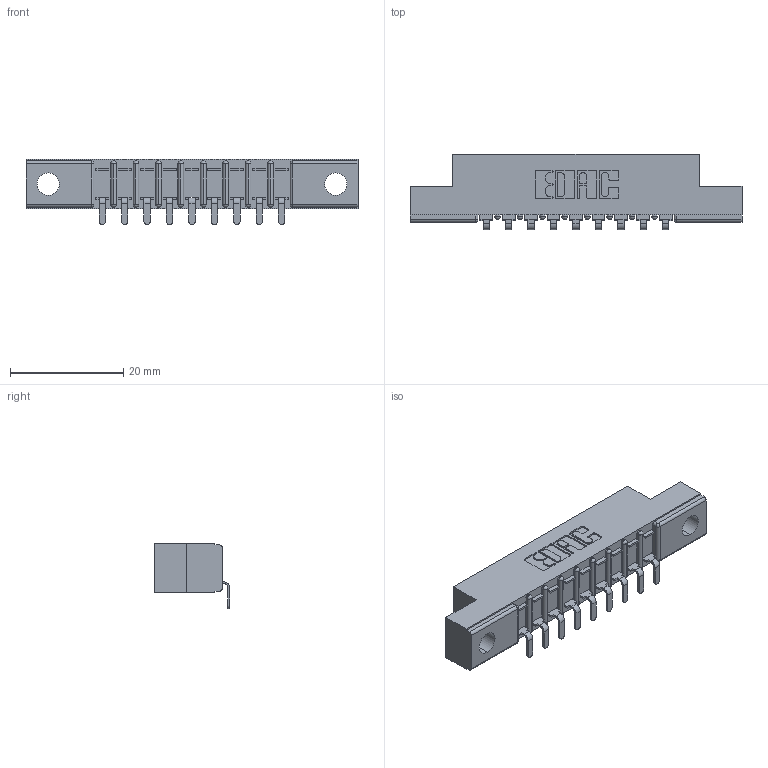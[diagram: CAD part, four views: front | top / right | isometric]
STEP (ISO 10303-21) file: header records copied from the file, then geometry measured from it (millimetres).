
FILE_DESCRIPTION (( 'STEP AP203' ), '1' );
FILE_NAME ('357-009-553-104.STEP', '2019-09-16T18:07:34', ( '' ), ( '' ), 'SwSTEP 2.0', 'SolidWorks 2016', '' );
FILE_SCHEMA (( 'CONFIG_CONTROL_DESIGN' ));
Length unit declared in the file: inch
Products named in the file (3): 307-290-002_553; 307 Part_.156 Dia Mounting Holes; 357-009-553-104
Assembly tree (10 placements, depth 2):
  357-009-553-104
    307 Part_.156 Dia Mounting Holes
    307-290-002_553  x9
Bounding box: 58.67 x 13.32 x 11.51 mm (x, y, z)
Volume: 3760.7 mm3; surface area: 6010.8 mm2
Topology: 10 solids, 10 shells, 844 faces, 2555 edges, 1674 vertices
Faces by surface type: plane 507, cylinder 317, sphere 20
Entity records: 13056 total; most frequent: CARTESIAN_POINT 2202, ORIENTED_EDGE 2190, DIRECTION 2147, EDGE_CURVE 1095, LINE 829, VECTOR 829, VERTEX_POINT 714, AXIS2_PLACEMENT_3D 659
